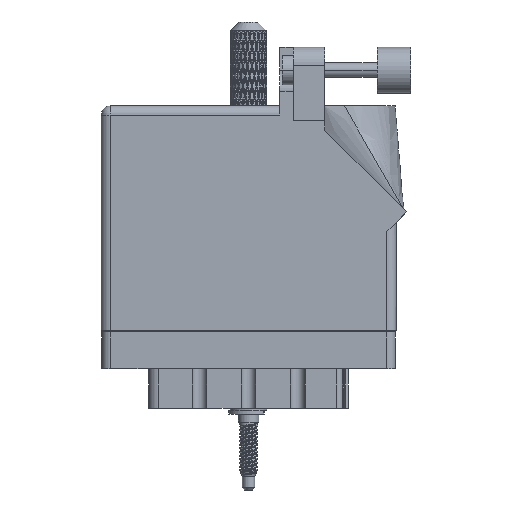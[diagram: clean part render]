
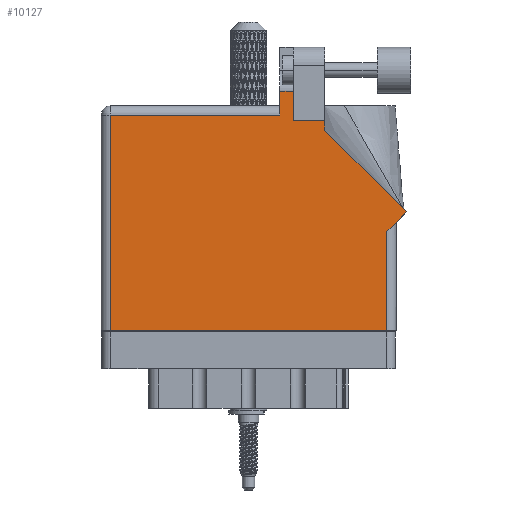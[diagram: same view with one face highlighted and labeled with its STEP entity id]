
A CAD part, front view. The second image highlights one B-rep face of the part: STEP entity #10127.
In plain terms, the highlighted face is planar.
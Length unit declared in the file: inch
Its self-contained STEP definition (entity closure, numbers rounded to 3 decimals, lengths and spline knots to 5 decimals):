
#251 = VECTOR ( 'NONE', #46596, 39.37008 ) ;
#818 = VERTEX_POINT ( 'NONE', #11335 ) ;
#1837 = LINE ( 'NONE', #85132, #40882 ) ;
#2127 = ORIENTED_EDGE ( 'NONE', *, *, #51172, .T. ) ;
#2503 = DIRECTION ( 'NONE',  ( -1., 0., 0. ) ) ;
#3307 = CARTESIAN_POINT ( 'NONE',  ( 2.01, 0.737, 0. ) ) ;
#5054 = AXIS2_PLACEMENT_3D ( 'NONE', #75159, #50631, #33553 ) ;
#5196 = DIRECTION ( 'NONE',  ( 0., 1., 0. ) ) ;
#7735 = EDGE_CURVE ( 'NONE', #25650, #85677, #35233, .T. ) ;
#9165 = CARTESIAN_POINT ( 'NONE',  ( 0.062, 0., 0. ) ) ;
#9323 = CARTESIAN_POINT ( 'NONE',  ( 1.217, 1.53, 0. ) ) ;
#9680 = DIRECTION ( 'NONE',  ( 0., -1., 0. ) ) ;
#10127 = ADVANCED_FACE ( 'NONE', ( #24482 ), #74812, .F. ) ;
#11335 = CARTESIAN_POINT ( 'NONE',  ( 0.062, 1.468, 0. ) ) ;
#11361 = CARTESIAN_POINT ( 'NONE',  ( 1.524, 1.43, 0. ) ) ;
#11785 = CARTESIAN_POINT ( 'NONE',  ( 0.062, 0., 0. ) ) ;
#12638 = VECTOR ( 'NONE', #107299, 39.37008 ) ;
#12796 = ORIENTED_EDGE ( 'NONE', *, *, #97121, .T. ) ;
#12959 = VERTEX_POINT ( 'NONE', #106955 ) ;
#13618 = CARTESIAN_POINT ( 'NONE',  ( 1.948, 0.675, 0. ) ) ;
#14188 = DIRECTION ( 'NONE',  ( -1., 0., 0. ) ) ;
#14629 = CARTESIAN_POINT ( 'NONE',  ( 0., 0., 0. ) ) ;
#16778 = VECTOR ( 'NONE', #5196, 39.37008 ) ;
#19927 = VERTEX_POINT ( 'NONE', #42717 ) ;
#20265 = DIRECTION ( 'NONE',  ( -1., 0., 0. ) ) ;
#21011 = VERTEX_POINT ( 'NONE', #57333 ) ;
#21926 = ORIENTED_EDGE ( 'NONE', *, *, #25684, .T. ) ;
#22192 = VECTOR ( 'NONE', #20265, 39.37008 ) ;
#22216 = CARTESIAN_POINT ( 'NONE',  ( 1.948, 0.737, 0. ) ) ;
#24482 = FACE_OUTER_BOUND ( 'NONE', #59732, .T. ) ;
#25111 = ORIENTED_EDGE ( 'NONE', *, *, #38577, .T. ) ;
#25650 = VERTEX_POINT ( 'NONE', #11361 ) ;
#25658 = LINE ( 'NONE', #14629, #12638 ) ;
#25684 = EDGE_CURVE ( 'NONE', #78687, #21011, #39714, .T. ) ;
#26975 = LINE ( 'NONE', #89156, #58090 ) ;
#28853 = VECTOR ( 'NONE', #9680, 39.37008 ) ;
#29361 = VECTOR ( 'NONE', #70811, 39.37008 ) ;
#33553 = DIRECTION ( 'NONE',  ( -1., 0., 0. ) ) ;
#35233 = LINE ( 'NONE', #68556, #22192 ) ;
#36893 = ORIENTED_EDGE ( 'NONE', *, *, #87178, .T. ) ;
#37810 = DIRECTION ( 'NONE',  ( -0.707, 0.707, 0. ) ) ;
#38577 = EDGE_CURVE ( 'NONE', #21011, #80095, #104434, .T. ) ;
#39714 = LINE ( 'NONE', #3307, #29361 ) ;
#40882 = VECTOR ( 'NONE', #2503, 39.37008 ) ;
#40902 = ORIENTED_EDGE ( 'NONE', *, *, #43059, .T. ) ;
#41112 = VECTOR ( 'NONE', #37810, 39.37008 ) ;
#41715 = CARTESIAN_POINT ( 'NONE',  ( 1.524, 1.36442, 0. ) ) ;
#42207 = VECTOR ( 'NONE', #82925, 39.37008 ) ;
#42717 = CARTESIAN_POINT ( 'NONE',  ( 1.311, 1.6315, 0. ) ) ;
#43059 = EDGE_CURVE ( 'NONE', #68781, #99136, #52279, .T. ) ;
#45401 = LINE ( 'NONE', #54957, #16778 ) ;
#46596 = DIRECTION ( 'NONE',  ( 0., 1., 0. ) ) ;
#47084 = CARTESIAN_POINT ( 'NONE',  ( 1.524, 1.36442, 0. ) ) ;
#47711 = CARTESIAN_POINT ( 'NONE',  ( 1.311, 1.43, 0. ) ) ;
#50631 = DIRECTION ( 'NONE',  ( 0., 0., -1. ) ) ;
#51172 = EDGE_CURVE ( 'NONE', #19927, #68781, #26975, .T. ) ;
#52279 = LINE ( 'NONE', #9323, #28853 ) ;
#52604 = LINE ( 'NONE', #41715, #42207 ) ;
#54957 = CARTESIAN_POINT ( 'NONE',  ( 1.311, 1.43, 0. ) ) ;
#55185 = ORIENTED_EDGE ( 'NONE', *, *, #71780, .T. ) ;
#57333 = CARTESIAN_POINT ( 'NONE',  ( 2.08071, 0.80771, 0. ) ) ;
#58090 = VECTOR ( 'NONE', #14188, 39.37008 ) ;
#59385 = EDGE_CURVE ( 'NONE', #80095, #25650, #52604, .T. ) ;
#59732 = EDGE_LOOP ( 'NONE', ( #99900, #2127, #40902, #36893, #55185, #12796, #84954, #21926, #25111, #88104, #106125 ) ) ;
#63246 = VECTOR ( 'NONE', #85319, 39.37008 ) ;
#65869 = LINE ( 'NONE', #11785, #63246 ) ;
#68556 = CARTESIAN_POINT ( 'NONE',  ( 1.524, 1.43, 0. ) ) ;
#68781 = VERTEX_POINT ( 'NONE', #83172 ) ;
#70021 = EDGE_CURVE ( 'NONE', #85677, #19927, #45401, .T. ) ;
#70811 = DIRECTION ( 'NONE',  ( 0.707, 0.707, 0. ) ) ;
#71780 = EDGE_CURVE ( 'NONE', #818, #92441, #65869, .T. ) ;
#74812 = PLANE ( 'NONE',  #5054 ) ;
#75159 = CARTESIAN_POINT ( 'NONE',  ( 0., 1.53, 0. ) ) ;
#78687 = VERTEX_POINT ( 'NONE', #13618 ) ;
#80095 = VERTEX_POINT ( 'NONE', #47084 ) ;
#80155 = CARTESIAN_POINT ( 'NONE',  ( 2.08071, 0.80771, 0. ) ) ;
#82925 = DIRECTION ( 'NONE',  ( 0., 1., 0. ) ) ;
#83172 = CARTESIAN_POINT ( 'NONE',  ( 1.217, 1.6315, 0. ) ) ;
#84954 = ORIENTED_EDGE ( 'NONE', *, *, #88839, .T. ) ;
#85132 = CARTESIAN_POINT ( 'NONE',  ( 0., 1.468, 0. ) ) ;
#85319 = DIRECTION ( 'NONE',  ( 0., -1., 0. ) ) ;
#85677 = VERTEX_POINT ( 'NONE', #47711 ) ;
#87178 = EDGE_CURVE ( 'NONE', #99136, #818, #1837, .T. ) ;
#88104 = ORIENTED_EDGE ( 'NONE', *, *, #59385, .T. ) ;
#88839 = EDGE_CURVE ( 'NONE', #12959, #78687, #89702, .T. ) ;
#89156 = CARTESIAN_POINT ( 'NONE',  ( 1.64177, 1.6315, 0. ) ) ;
#89702 = LINE ( 'NONE', #22216, #251 ) ;
#92441 = VERTEX_POINT ( 'NONE', #9165 ) ;
#97121 = EDGE_CURVE ( 'NONE', #92441, #12959, #25658, .T. ) ;
#97831 = CARTESIAN_POINT ( 'NONE',  ( 1.217, 1.468, 0. ) ) ;
#99136 = VERTEX_POINT ( 'NONE', #97831 ) ;
#99900 = ORIENTED_EDGE ( 'NONE', *, *, #70021, .T. ) ;
#104434 = LINE ( 'NONE', #80155, #41112 ) ;
#106125 = ORIENTED_EDGE ( 'NONE', *, *, #7735, .T. ) ;
#106955 = CARTESIAN_POINT ( 'NONE',  ( 1.948, 0., 0. ) ) ;
#107299 = DIRECTION ( 'NONE',  ( 1., 0., 0. ) ) ;
